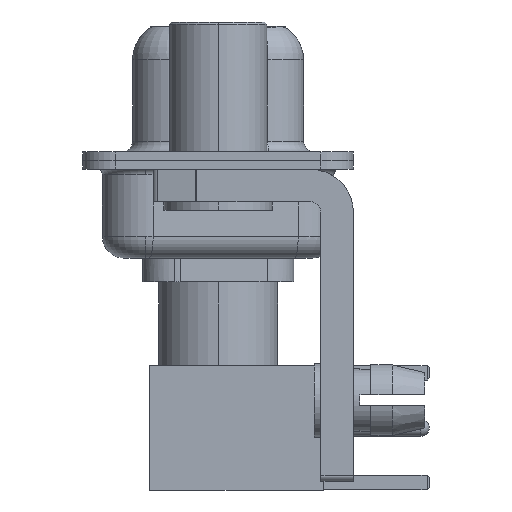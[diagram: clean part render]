
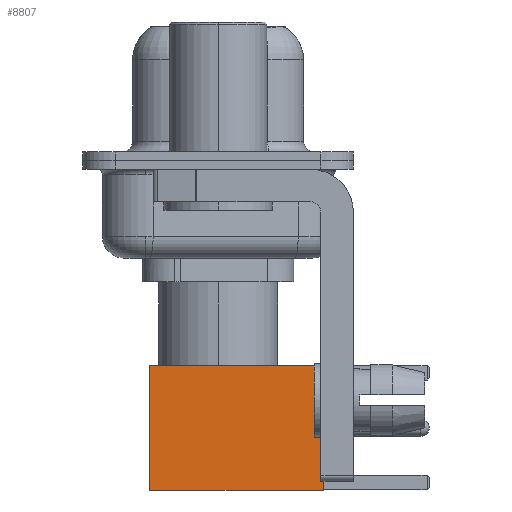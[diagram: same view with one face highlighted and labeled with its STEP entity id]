
A CAD part, left-side view. The second image highlights one B-rep face of the part: STEP entity #8807.
In plain terms, the highlighted face is planar.
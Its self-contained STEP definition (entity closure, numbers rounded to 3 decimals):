
#86 = EDGE_CURVE ( 'NONE', #11915, #4653, #14206, .T. ) ;
#1106 = EDGE_CURVE ( 'NONE', #11740, #11915, #12319, .T. ) ;
#1600 = CARTESIAN_POINT ( 'NONE',  ( 0., 2.875, 8. ) ) ;
#2232 = EDGE_CURVE ( 'NONE', #19890, #4653, #4430, .T. ) ;
#2329 = CARTESIAN_POINT ( 'NONE',  ( 2.875, 2.875, 8. ) ) ;
#2777 = DIRECTION ( 'NONE',  ( -1., 0., 0. ) ) ;
#3050 = AXIS2_PLACEMENT_3D ( 'NONE', #10072, #17814, #3535 ) ;
#3535 = DIRECTION ( 'NONE',  ( 0., 0., 1. ) ) ;
#4163 = VECTOR ( 'NONE', #2777, 1000. ) ;
#4175 = ORIENTED_EDGE ( 'NONE', *, *, #2232, .T. ) ;
#4430 = LINE ( 'NONE', #12409, #9784 ) ;
#4653 = VERTEX_POINT ( 'NONE', #7473 ) ;
#4804 = LINE ( 'NONE', #16026, #10125 ) ;
#4878 = CARTESIAN_POINT ( 'NONE',  ( -2.875, 2.875, 8. ) ) ;
#5068 = PLANE ( 'NONE',  #3050 ) ;
#5329 = DIRECTION ( 'NONE',  ( 0., 0., -1. ) ) ;
#5594 = CARTESIAN_POINT ( 'NONE',  ( 2.875, 2.875, 0. ) ) ;
#5781 = ORIENTED_EDGE ( 'NONE', *, *, #19281, .T. ) ;
#6908 = FACE_OUTER_BOUND ( 'NONE', #11873, .T. ) ;
#7473 = CARTESIAN_POINT ( 'NONE',  ( -2.875, 2.875, 0. ) ) ;
#7985 = DIRECTION ( 'NONE',  ( 0., 0., -1. ) ) ;
#8807 = ADVANCED_FACE ( 'NONE', ( #6908 ), #5068, .T. ) ;
#9784 = VECTOR ( 'NONE', #18618, 1000. ) ;
#10072 = CARTESIAN_POINT ( 'NONE',  ( 2.875, 2.875, 0. ) ) ;
#10125 = VECTOR ( 'NONE', #7985, 1000. ) ;
#10706 = VECTOR ( 'NONE', #5329, 1000. ) ;
#11740 = VERTEX_POINT ( 'NONE', #2329 ) ;
#11873 = EDGE_LOOP ( 'NONE', ( #5781, #4175, #19224, #16874 ) ) ;
#11915 = VERTEX_POINT ( 'NONE', #4878 ) ;
#12319 = LINE ( 'NONE', #1600, #4163 ) ;
#12409 = CARTESIAN_POINT ( 'NONE',  ( 0., 2.875, 0. ) ) ;
#14206 = LINE ( 'NONE', #17468, #10706 ) ;
#16026 = CARTESIAN_POINT ( 'NONE',  ( 2.875, 2.875, 0. ) ) ;
#16874 = ORIENTED_EDGE ( 'NONE', *, *, #1106, .F. ) ;
#17468 = CARTESIAN_POINT ( 'NONE',  ( -2.875, 2.875, 0. ) ) ;
#17814 = DIRECTION ( 'NONE',  ( 0., 1., 0. ) ) ;
#18618 = DIRECTION ( 'NONE',  ( -1., 0., 0. ) ) ;
#19224 = ORIENTED_EDGE ( 'NONE', *, *, #86, .F. ) ;
#19281 = EDGE_CURVE ( 'NONE', #11740, #19890, #4804, .T. ) ;
#19890 = VERTEX_POINT ( 'NONE', #5594 ) ;
